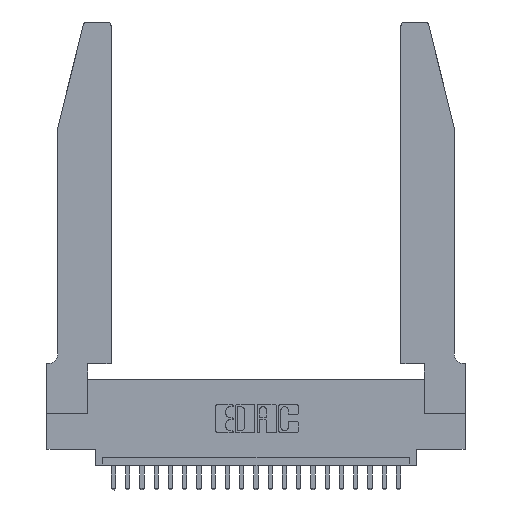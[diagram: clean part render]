
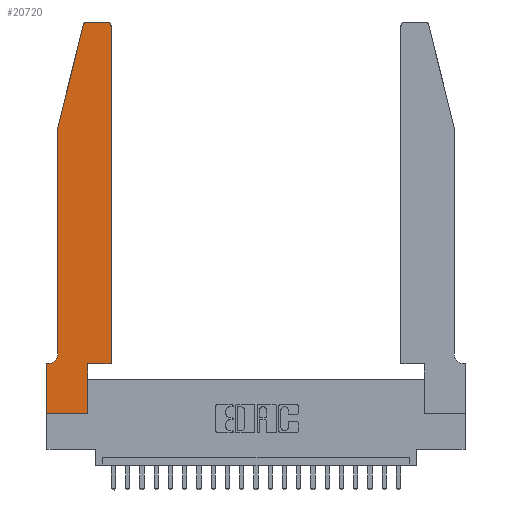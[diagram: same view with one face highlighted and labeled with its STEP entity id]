
A CAD part, top view. The second image highlights one B-rep face of the part: STEP entity #20720.
In plain terms, the highlighted planar face has unit normal (0, 0, 1).
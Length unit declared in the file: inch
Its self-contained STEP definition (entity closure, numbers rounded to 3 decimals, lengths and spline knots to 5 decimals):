
#136 = CIRCLE ( 'NONE', #6911, 0.03 ) ;
#1213 = VERTEX_POINT ( 'NONE', #4890 ) ;
#1773 = DIRECTION ( 'NONE',  ( 0., -1., 0. ) ) ;
#1803 = VECTOR ( 'NONE', #18761, 39.37008 ) ;
#1910 = CARTESIAN_POINT ( 'NONE',  ( 0.4205, 2.75, 0.37 ) ) ;
#2616 = CARTESIAN_POINT ( 'NONE',  ( 0.284, 2.75, 0.37 ) ) ;
#2653 = EDGE_CURVE ( 'NONE', #11121, #1213, #20343, .T. ) ;
#3375 = CARTESIAN_POINT ( 'NONE',  ( 0.4505, 0.35, 0.37 ) ) ;
#3459 = EDGE_CURVE ( 'NONE', #15939, #14374, #16029, .T. ) ;
#3608 = CARTESIAN_POINT ( 'NONE',  ( 0., 0., 0.37 ) ) ;
#3706 = CARTESIAN_POINT ( 'NONE',  ( 0.2865, 0., 0.37 ) ) ;
#3912 = DIRECTION ( 'NONE',  ( 0., -1., 0. ) ) ;
#4114 = DIRECTION ( 'NONE',  ( 0., 0., 1. ) ) ;
#4153 = VECTOR ( 'NONE', #1773, 39.37008 ) ;
#4277 = EDGE_CURVE ( 'NONE', #21282, #11464, #17697, .T. ) ;
#4317 = ORIENTED_EDGE ( 'NONE', *, *, #4277, .T. ) ;
#4363 = CARTESIAN_POINT ( 'NONE',  ( 0.0755, 2., 0.37 ) ) ;
#4719 = ORIENTED_EDGE ( 'NONE', *, *, #16683, .T. ) ;
#4890 = CARTESIAN_POINT ( 'NONE',  ( 0.4505, 2.72, 0.37 ) ) ;
#4909 = DIRECTION ( 'NONE',  ( 0., 1., 0. ) ) ;
#5196 = DIRECTION ( 'NONE',  ( 0., 0., 1. ) ) ;
#5331 = VERTEX_POINT ( 'NONE', #10828 ) ;
#5408 = CARTESIAN_POINT ( 'NONE',  ( 0.25487, 2.72718, 0.37 ) ) ;
#5435 = ORIENTED_EDGE ( 'NONE', *, *, #18453, .T. ) ;
#5446 = VECTOR ( 'NONE', #10218, 39.37008 ) ;
#5769 = EDGE_CURVE ( 'NONE', #8943, #10646, #6784, .T. ) ;
#5910 = EDGE_LOOP ( 'NONE', ( #8623, #5435, #7997, #16608, #11430, #10179, #13909, #21313, #4317, #13948, #20836, #4719 ) ) ;
#6077 = LINE ( 'NONE', #22447, #1803 ) ;
#6784 = LINE ( 'NONE', #17763, #15650 ) ;
#6911 = AXIS2_PLACEMENT_3D ( 'NONE', #22276, #4114, #7761 ) ;
#7460 = EDGE_CURVE ( 'NONE', #19095, #22142, #12095, .T. ) ;
#7761 = DIRECTION ( 'NONE',  ( 1., 0., 0. ) ) ;
#7997 = ORIENTED_EDGE ( 'NONE', *, *, #22697, .T. ) ;
#8502 = FACE_OUTER_BOUND ( 'NONE', #5910, .T. ) ;
#8623 = ORIENTED_EDGE ( 'NONE', *, *, #3459, .T. ) ;
#8777 = CARTESIAN_POINT ( 'NONE',  ( 0., 0.35, 0.37 ) ) ;
#8943 = VERTEX_POINT ( 'NONE', #8777 ) ;
#9043 = VECTOR ( 'NONE', #4909, 39.37008 ) ;
#9102 = DIRECTION ( 'NONE',  ( 1., 0., 0. ) ) ;
#9228 = CARTESIAN_POINT ( 'NONE',  ( 0.0055, 0.42, 0.37 ) ) ;
#9347 = CARTESIAN_POINT ( 'NONE',  ( 0.0755, 2., 0.37 ) ) ;
#9395 = DIRECTION ( 'NONE',  ( -1., 0., 0. ) ) ;
#9692 = CARTESIAN_POINT ( 'NONE',  ( 0.0755, 0.35, 0.37 ) ) ;
#9840 = EDGE_CURVE ( 'NONE', #22142, #5331, #10240, .T. ) ;
#10179 = ORIENTED_EDGE ( 'NONE', *, *, #16127, .T. ) ;
#10218 = DIRECTION ( 'NONE',  ( -1., 0., 0. ) ) ;
#10240 = CIRCLE ( 'NONE', #10536, 0.07 ) ;
#10536 = AXIS2_PLACEMENT_3D ( 'NONE', #9228, #22040, #9395 ) ;
#10646 = VERTEX_POINT ( 'NONE', #17859 ) ;
#10828 = CARTESIAN_POINT ( 'NONE',  ( 0.0055, 0.35, 0.37 ) ) ;
#11066 = AXIS2_PLACEMENT_3D ( 'NONE', #13050, #16592, #9102 ) ;
#11121 = VERTEX_POINT ( 'NONE', #3375 ) ;
#11430 = ORIENTED_EDGE ( 'NONE', *, *, #9840, .T. ) ;
#11460 = LINE ( 'NONE', #21462, #21492 ) ;
#11464 = VERTEX_POINT ( 'NONE', #15931 ) ;
#11764 = CARTESIAN_POINT ( 'NONE',  ( 0.2605, 2.75, 0.37 ) ) ;
#12095 = LINE ( 'NONE', #9347, #4153 ) ;
#12624 = CIRCLE ( 'NONE', #16582, 0.03 ) ;
#12764 = CARTESIAN_POINT ( 'NONE',  ( 0.4505, 0.35, 0.37 ) ) ;
#13028 = VECTOR ( 'NONE', #17906, 39.37008 ) ;
#13050 = CARTESIAN_POINT ( 'NONE',  ( 0., 0.35, 0.37 ) ) ;
#13717 = EDGE_CURVE ( 'NONE', #10646, #21282, #17236, .T. ) ;
#13892 = CARTESIAN_POINT ( 'NONE',  ( 0.2865, 0.35, 0.37 ) ) ;
#13909 = ORIENTED_EDGE ( 'NONE', *, *, #5769, .T. ) ;
#13948 = ORIENTED_EDGE ( 'NONE', *, *, #18364, .T. ) ;
#14374 = VERTEX_POINT ( 'NONE', #2616 ) ;
#14528 = DIRECTION ( 'NONE',  ( 0., 1., 0. ) ) ;
#15650 = VECTOR ( 'NONE', #3912, 39.37008 ) ;
#15931 = CARTESIAN_POINT ( 'NONE',  ( 0.2865, 0.35, 0.37 ) ) ;
#15939 = VERTEX_POINT ( 'NONE', #1910 ) ;
#16029 = LINE ( 'NONE', #11764, #5446 ) ;
#16118 = CARTESIAN_POINT ( 'NONE',  ( 0.284, 2.72, 0.37 ) ) ;
#16127 = EDGE_CURVE ( 'NONE', #5331, #8943, #20480, .T. ) ;
#16427 = PLANE ( 'NONE',  #11066 ) ;
#16582 = AXIS2_PLACEMENT_3D ( 'NONE', #16118, #5196, #23590 ) ;
#16592 = DIRECTION ( 'NONE',  ( 0., 0., 1. ) ) ;
#16608 = ORIENTED_EDGE ( 'NONE', *, *, #7460, .T. ) ;
#16683 = EDGE_CURVE ( 'NONE', #1213, #15939, #136, .T. ) ;
#17236 = LINE ( 'NONE', #3608, #21496 ) ;
#17697 = LINE ( 'NONE', #13892, #9043 ) ;
#17763 = CARTESIAN_POINT ( 'NONE',  ( 0., 0., 0.37 ) ) ;
#17859 = CARTESIAN_POINT ( 'NONE',  ( 0., 0., 0.37 ) ) ;
#17906 = DIRECTION ( 'NONE',  ( -1., 0., 0. ) ) ;
#18364 = EDGE_CURVE ( 'NONE', #11464, #11121, #11460, .T. ) ;
#18371 = VECTOR ( 'NONE', #14528, 39.37008 ) ;
#18453 = EDGE_CURVE ( 'NONE', #14374, #18925, #12624, .T. ) ;
#18761 = DIRECTION ( 'NONE',  ( -0.239, -0.971, 0. ) ) ;
#18925 = VERTEX_POINT ( 'NONE', #5408 ) ;
#19095 = VERTEX_POINT ( 'NONE', #4363 ) ;
#19876 = DIRECTION ( 'NONE',  ( 1., 0., 0. ) ) ;
#20343 = LINE ( 'NONE', #12764, #18371 ) ;
#20480 = LINE ( 'NONE', #9692, #13028 ) ;
#20720 = ADVANCED_FACE ( 'NONE', ( #8502 ), #16427, .T. ) ;
#20836 = ORIENTED_EDGE ( 'NONE', *, *, #2653, .T. ) ;
#21282 = VERTEX_POINT ( 'NONE', #3706 ) ;
#21313 = ORIENTED_EDGE ( 'NONE', *, *, #13717, .T. ) ;
#21462 = CARTESIAN_POINT ( 'NONE',  ( 0.4505, 0.35, 0.37 ) ) ;
#21492 = VECTOR ( 'NONE', #19876, 39.37008 ) ;
#21496 = VECTOR ( 'NONE', #23547, 39.37008 ) ;
#22040 = DIRECTION ( 'NONE',  ( 0., 0., -1. ) ) ;
#22142 = VERTEX_POINT ( 'NONE', #22477 ) ;
#22276 = CARTESIAN_POINT ( 'NONE',  ( 0.4205, 2.72, 0.37 ) ) ;
#22447 = CARTESIAN_POINT ( 'NONE',  ( 0.0755, 2., 0.37 ) ) ;
#22477 = CARTESIAN_POINT ( 'NONE',  ( 0.0755, 0.42, 0.37 ) ) ;
#22697 = EDGE_CURVE ( 'NONE', #18925, #19095, #6077, .T. ) ;
#23547 = DIRECTION ( 'NONE',  ( 1., 0., 0. ) ) ;
#23590 = DIRECTION ( 'NONE',  ( 1., 0., 0. ) ) ;
